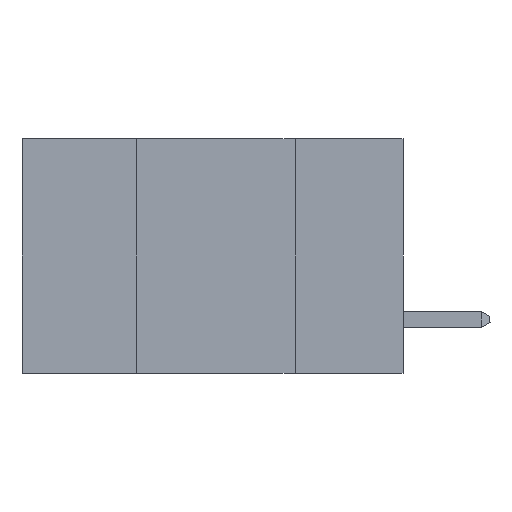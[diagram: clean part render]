
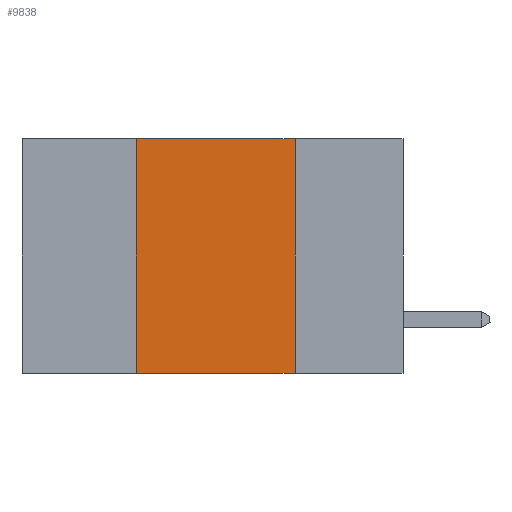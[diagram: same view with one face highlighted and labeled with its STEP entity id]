
A CAD part, left-side view. The second image highlights one B-rep face of the part: STEP entity #9838.
In plain terms, the highlighted planar face has unit normal (-1, 0, 0).
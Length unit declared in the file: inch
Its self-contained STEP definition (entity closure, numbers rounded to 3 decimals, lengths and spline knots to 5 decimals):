
#186 = CARTESIAN_POINT ( 'NONE',  ( 0., 0.42, 0. ) ) ;
#190 = CARTESIAN_POINT ( 'NONE',  ( 0., 0.6, -0.37 ) ) ;
#278 = DIRECTION ( 'NONE',  ( 0., -1., 0. ) ) ;
#309 = CARTESIAN_POINT ( 'NONE',  ( 0., 0.42, 0. ) ) ;
#407 = DIRECTION ( 'NONE',  ( 0., 0., 1. ) ) ;
#1124 = CARTESIAN_POINT ( 'NONE',  ( 0., 0.42, -0.37 ) ) ;
#2725 = VERTEX_POINT ( 'NONE', #13371 ) ;
#3591 = ORIENTED_EDGE ( 'NONE', *, *, #4523, .F. ) ;
#4099 = LINE ( 'NONE', #309, #6699 ) ;
#4209 = DIRECTION ( 'NONE',  ( 1., 0., 0. ) ) ;
#4523 = EDGE_CURVE ( 'NONE', #10584, #5352, #4099, .T. ) ;
#4585 = EDGE_CURVE ( 'NONE', #5352, #2725, #5489, .T. ) ;
#4619 = EDGE_LOOP ( 'NONE', ( #6349, #6988, #3591, #12412 ) ) ;
#4817 = CARTESIAN_POINT ( 'NONE',  ( 0., 0.6, 0. ) ) ;
#4912 = EDGE_CURVE ( 'NONE', #10584, #11478, #14036, .T. ) ;
#5352 = VERTEX_POINT ( 'NONE', #186 ) ;
#5412 = PLANE ( 'NONE',  #7787 ) ;
#5489 = LINE ( 'NONE', #4817, #12146 ) ;
#6082 = DIRECTION ( 'NONE',  ( 0., 0., -1. ) ) ;
#6124 = DIRECTION ( 'NONE',  ( 0., -1., 0. ) ) ;
#6349 = ORIENTED_EDGE ( 'NONE', *, *, #10266, .F. ) ;
#6699 = VECTOR ( 'NONE', #407, 39.37008 ) ;
#6988 = ORIENTED_EDGE ( 'NONE', *, *, #4585, .F. ) ;
#7575 = VECTOR ( 'NONE', #278, 39.37008 ) ;
#7787 = AXIS2_PLACEMENT_3D ( 'NONE', #12073, #4209, #12120 ) ;
#7855 = LINE ( 'NONE', #13748, #9481 ) ;
#9481 = VECTOR ( 'NONE', #6082, 39.37008 ) ;
#9833 = FACE_OUTER_BOUND ( 'NONE', #4619, .T. ) ;
#9838 = ADVANCED_FACE ( 'NONE', ( #9833 ), #5412, .F. ) ;
#10266 = EDGE_CURVE ( 'NONE', #2725, #11478, #7855, .T. ) ;
#10584 = VERTEX_POINT ( 'NONE', #1124 ) ;
#11173 = CARTESIAN_POINT ( 'NONE',  ( 0., 0.17, -0.37 ) ) ;
#11478 = VERTEX_POINT ( 'NONE', #11173 ) ;
#12073 = CARTESIAN_POINT ( 'NONE',  ( 0., 0.6, 0. ) ) ;
#12120 = DIRECTION ( 'NONE',  ( 0., 0., -1. ) ) ;
#12146 = VECTOR ( 'NONE', #6124, 39.37008 ) ;
#12412 = ORIENTED_EDGE ( 'NONE', *, *, #4912, .T. ) ;
#13371 = CARTESIAN_POINT ( 'NONE',  ( 0., 0.17, 0. ) ) ;
#13748 = CARTESIAN_POINT ( 'NONE',  ( 0., 0.17, 0. ) ) ;
#14036 = LINE ( 'NONE', #190, #7575 ) ;
